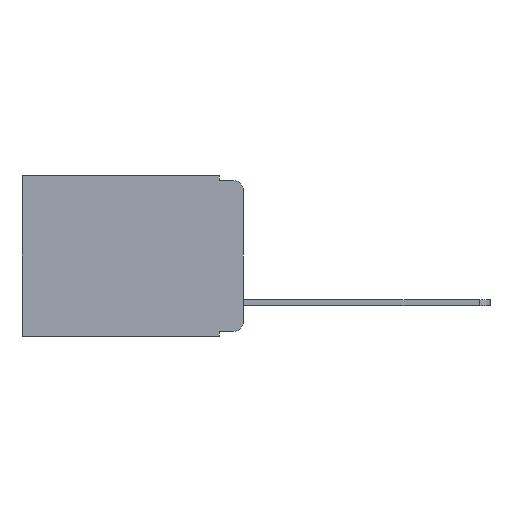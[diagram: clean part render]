
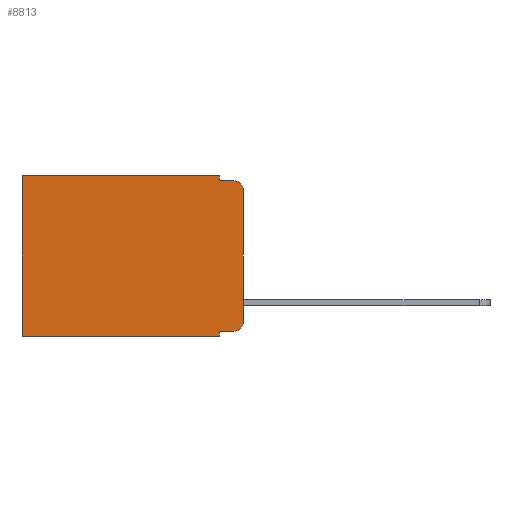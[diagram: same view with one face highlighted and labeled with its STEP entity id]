
A CAD part, left-side view. The second image highlights one B-rep face of the part: STEP entity #8813.
In plain terms, the highlighted planar face has unit normal (-1, 0, 0).
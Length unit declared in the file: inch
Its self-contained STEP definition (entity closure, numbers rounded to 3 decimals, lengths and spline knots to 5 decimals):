
#169 = LINE ( 'NONE', #12162, #4012 ) ;
#645 = CARTESIAN_POINT ( 'NONE',  ( 0.298, 0.473, 0. ) ) ;
#744 = CARTESIAN_POINT ( 'NONE',  ( 0.298, 0.473, -0.343 ) ) ;
#759 = VERTEX_POINT ( 'NONE', #16928 ) ;
#1109 = VERTEX_POINT ( 'NONE', #12513 ) ;
#1303 = EDGE_CURVE ( 'NONE', #2720, #759, #12068, .T. ) ;
#1596 = CARTESIAN_POINT ( 'NONE',  ( 0.298, 0.473, 0. ) ) ;
#2081 = DIRECTION ( 'NONE',  ( 0., 0., -1. ) ) ;
#2177 = DIRECTION ( 'NONE',  ( 0., 1., 0. ) ) ;
#2567 = DIRECTION ( 'NONE',  ( 0., 0., -1. ) ) ;
#2720 = VERTEX_POINT ( 'NONE', #10678 ) ;
#2883 = CARTESIAN_POINT ( 'NONE',  ( 0.298, 0.02, -0.333 ) ) ;
#2897 = CARTESIAN_POINT ( 'NONE',  ( 0.298, 0., 0. ) ) ;
#3061 = ORIENTED_EDGE ( 'NONE', *, *, #6640, .F. ) ;
#3064 = AXIS2_PLACEMENT_3D ( 'NONE', #14772, #7161, #16049 ) ;
#3142 = VECTOR ( 'NONE', #2177, 39.37008 ) ;
#3483 = DIRECTION ( 'NONE',  ( 0., -1., 0. ) ) ;
#3538 = VECTOR ( 'NONE', #2567, 39.37008 ) ;
#3696 = CARTESIAN_POINT ( 'NONE',  ( 0.298, 0.051, -0.333 ) ) ;
#4012 = VECTOR ( 'NONE', #13412, 39.37008 ) ;
#4016 = AXIS2_PLACEMENT_3D ( 'NONE', #2897, #15997, #8417 ) ;
#4487 = DIRECTION ( 'NONE',  ( 0., 0., -1. ) ) ;
#4852 = CARTESIAN_POINT ( 'NONE',  ( 0.298, 0.051, -0.333 ) ) ;
#5070 = ORIENTED_EDGE ( 'NONE', *, *, #13883, .T. ) ;
#5495 = ORIENTED_EDGE ( 'NONE', *, *, #7375, .F. ) ;
#5922 = VERTEX_POINT ( 'NONE', #1596 ) ;
#5986 = VERTEX_POINT ( 'NONE', #12128 ) ;
#6640 = EDGE_CURVE ( 'NONE', #1109, #759, #15054, .T. ) ;
#6763 = LINE ( 'NONE', #11812, #9749 ) ;
#6789 = ORIENTED_EDGE ( 'NONE', *, *, #9634, .T. ) ;
#6983 = DIRECTION ( 'NONE',  ( 0., 0., -1. ) ) ;
#7113 = EDGE_LOOP ( 'NONE', ( #11173, #12384, #3061, #14953, #5070, #12771, #5495, #9024, #6789, #14764 ) ) ;
#7161 = DIRECTION ( 'NONE',  ( -1., 0., 0. ) ) ;
#7316 = VECTOR ( 'NONE', #2081, 39.37008 ) ;
#7375 = EDGE_CURVE ( 'NONE', #14300, #11597, #13226, .T. ) ;
#7646 = EDGE_CURVE ( 'NONE', #2720, #5986, #11861, .T. ) ;
#7847 = CARTESIAN_POINT ( 'NONE',  ( 0.298, 0.051, 0. ) ) ;
#8291 = AXIS2_PLACEMENT_3D ( 'NONE', #8560, #16070, #6983 ) ;
#8417 = DIRECTION ( 'NONE',  ( 0., 0., -1. ) ) ;
#8488 = VECTOR ( 'NONE', #4487, 39.37008 ) ;
#8511 = CARTESIAN_POINT ( 'NONE',  ( 0.298, 0., 0. ) ) ;
#8560 = CARTESIAN_POINT ( 'NONE',  ( 0.298, 0.02, -0.03 ) ) ;
#8813 = ADVANCED_FACE ( 'NONE', ( #13771 ), #10893, .F. ) ;
#8820 = EDGE_CURVE ( 'NONE', #13877, #5986, #9989, .T. ) ;
#9024 = ORIENTED_EDGE ( 'NONE', *, *, #10499, .F. ) ;
#9242 = EDGE_CURVE ( 'NONE', #17009, #1109, #10621, .T. ) ;
#9634 = EDGE_CURVE ( 'NONE', #15268, #13877, #16922, .T. ) ;
#9749 = VECTOR ( 'NONE', #13062, 39.37008 ) ;
#9989 = CIRCLE ( 'NONE', #3064, 0.02 ) ;
#10262 = CARTESIAN_POINT ( 'NONE',  ( 0.298, 0., -0.343 ) ) ;
#10499 = EDGE_CURVE ( 'NONE', #15268, #14300, #6763, .T. ) ;
#10621 = LINE ( 'NONE', #13131, #3538 ) ;
#10678 = CARTESIAN_POINT ( 'NONE',  ( 0.298, 0., -0.03 ) ) ;
#10888 = VECTOR ( 'NONE', #16742, 39.37008 ) ;
#10893 = PLANE ( 'NONE',  #4016 ) ;
#11173 = ORIENTED_EDGE ( 'NONE', *, *, #7646, .F. ) ;
#11597 = VERTEX_POINT ( 'NONE', #744 ) ;
#11812 = CARTESIAN_POINT ( 'NONE',  ( 0.298, 0.051, 0. ) ) ;
#11860 = CARTESIAN_POINT ( 'NONE',  ( 0.298, 0.051, -0.01 ) ) ;
#11861 = LINE ( 'NONE', #8511, #8488 ) ;
#12068 = CIRCLE ( 'NONE', #8291, 0.02 ) ;
#12128 = CARTESIAN_POINT ( 'NONE',  ( 0.298, 0., -0.313 ) ) ;
#12162 = CARTESIAN_POINT ( 'NONE',  ( 0.298, 0., 0. ) ) ;
#12384 = ORIENTED_EDGE ( 'NONE', *, *, #1303, .T. ) ;
#12513 = CARTESIAN_POINT ( 'NONE',  ( 0.298, 0.051, -0.01 ) ) ;
#12771 = ORIENTED_EDGE ( 'NONE', *, *, #13036, .T. ) ;
#13021 = CARTESIAN_POINT ( 'NONE',  ( 0.298, 0.051, -0.343 ) ) ;
#13036 = EDGE_CURVE ( 'NONE', #5922, #11597, #14050, .T. ) ;
#13062 = DIRECTION ( 'NONE',  ( 0., 0., -1. ) ) ;
#13131 = CARTESIAN_POINT ( 'NONE',  ( 0.298, 0.051, 0. ) ) ;
#13226 = LINE ( 'NONE', #10262, #3142 ) ;
#13412 = DIRECTION ( 'NONE',  ( 0., 1., 0. ) ) ;
#13562 = VECTOR ( 'NONE', #3483, 39.37008 ) ;
#13771 = FACE_OUTER_BOUND ( 'NONE', #7113, .T. ) ;
#13877 = VERTEX_POINT ( 'NONE', #2883 ) ;
#13883 = EDGE_CURVE ( 'NONE', #17009, #5922, #169, .T. ) ;
#14050 = LINE ( 'NONE', #645, #7316 ) ;
#14300 = VERTEX_POINT ( 'NONE', #13021 ) ;
#14764 = ORIENTED_EDGE ( 'NONE', *, *, #8820, .T. ) ;
#14772 = CARTESIAN_POINT ( 'NONE',  ( 0.298, 0.02, -0.313 ) ) ;
#14953 = ORIENTED_EDGE ( 'NONE', *, *, #9242, .F. ) ;
#15054 = LINE ( 'NONE', #11860, #10888 ) ;
#15268 = VERTEX_POINT ( 'NONE', #3696 ) ;
#15997 = DIRECTION ( 'NONE',  ( 1., 0., 0. ) ) ;
#16049 = DIRECTION ( 'NONE',  ( 0., 0., -1. ) ) ;
#16070 = DIRECTION ( 'NONE',  ( -1., 0., 0. ) ) ;
#16742 = DIRECTION ( 'NONE',  ( 0., -1., 0. ) ) ;
#16922 = LINE ( 'NONE', #4852, #13562 ) ;
#16928 = CARTESIAN_POINT ( 'NONE',  ( 0.298, 0.02, -0.01 ) ) ;
#17009 = VERTEX_POINT ( 'NONE', #7847 ) ;
